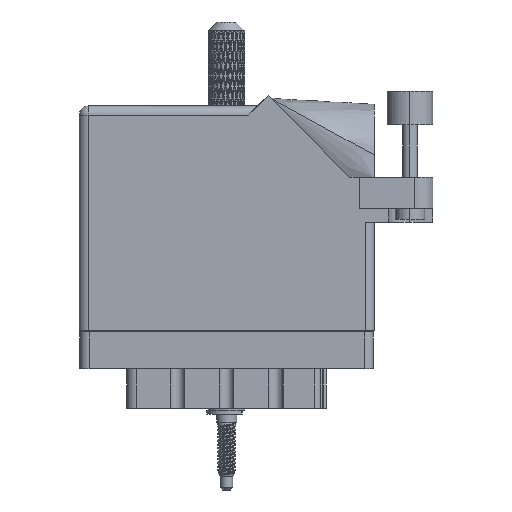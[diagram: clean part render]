
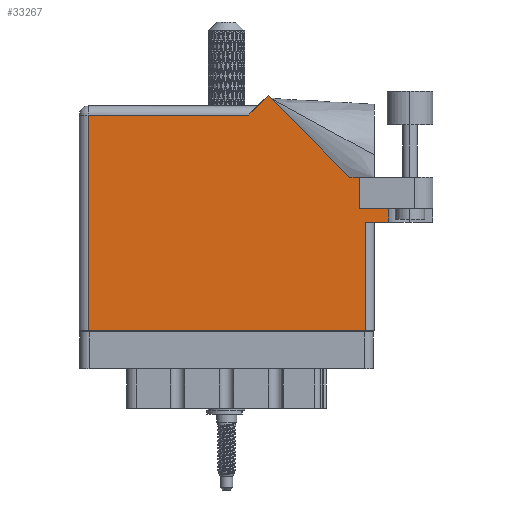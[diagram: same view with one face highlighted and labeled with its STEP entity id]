
A CAD part, front view. The second image highlights one B-rep face of the part: STEP entity #33267.
In plain terms, the highlighted face is planar.
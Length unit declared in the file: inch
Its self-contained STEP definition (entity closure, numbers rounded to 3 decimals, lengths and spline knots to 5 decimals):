
#1179 = FACE_OUTER_BOUND ( 'NONE', #18269, .T. ) ;
#2313 = VERTEX_POINT ( 'NONE', #89890 ) ;
#4279 = EDGE_CURVE ( 'NONE', #44404, #7908, #83758, .T. ) ;
#4425 = EDGE_CURVE ( 'NONE', #72469, #58199, #65546, .T. ) ;
#4754 = CARTESIAN_POINT ( 'NONE',  ( 1.91, 1.044, 0. ) ) ;
#7340 = ORIENTED_EDGE ( 'NONE', *, *, #96079, .T. ) ;
#7737 = EDGE_CURVE ( 'NONE', #39307, #41077, #88404, .T. ) ;
#7908 = VERTEX_POINT ( 'NONE', #36448 ) ;
#8182 = DIRECTION ( 'NONE',  ( -0.707, 0.707, 0. ) ) ;
#10214 = VERTEX_POINT ( 'NONE', #67415 ) ;
#15697 = LINE ( 'NONE', #27255, #35197 ) ;
#16125 = CARTESIAN_POINT ( 'NONE',  ( 1.84442, 1.044, 0. ) ) ;
#16187 = ORIENTED_EDGE ( 'NONE', *, *, #77938, .T. ) ;
#16701 = LINE ( 'NONE', #39897, #78989 ) ;
#18269 = EDGE_LOOP ( 'NONE', ( #16187, #7340, #90625, #33414, #62590, #101086, #53317, #51466, #72402, #36163, #60569 ) ) ;
#18594 = CARTESIAN_POINT ( 'NONE',  ( 1.91, 0.831, 0. ) ) ;
#19756 = VECTOR ( 'NONE', #8182, 39.37008 ) ;
#22445 = VECTOR ( 'NONE', #92384, 39.37008 ) ;
#25556 = EDGE_CURVE ( 'NONE', #72469, #82461, #66177, .T. ) ;
#27255 = CARTESIAN_POINT ( 'NONE',  ( 1.217, 1.53, 0. ) ) ;
#31715 = CARTESIAN_POINT ( 'NONE',  ( 2.01, 0.737, 0. ) ) ;
#31770 = VECTOR ( 'NONE', #35194, 39.37008 ) ;
#32326 = CARTESIAN_POINT ( 'NONE',  ( 2.1115, 0.831, 0. ) ) ;
#33267 = ADVANCED_FACE ( 'NONE', ( #1179 ), #75934, .F. ) ;
#33414 = ORIENTED_EDGE ( 'NONE', *, *, #39408, .F. ) ;
#33597 = DIRECTION ( 'NONE',  ( 0., 0., -1. ) ) ;
#33825 = DIRECTION ( 'NONE',  ( -0.707, -0.707, 0. ) ) ;
#35193 = CARTESIAN_POINT ( 'NONE',  ( 1.948, 0., 0. ) ) ;
#35194 = DIRECTION ( 'NONE',  ( -1., 0., 0. ) ) ;
#35197 = VECTOR ( 'NONE', #33825, 39.37008 ) ;
#36163 = ORIENTED_EDGE ( 'NONE', *, *, #59372, .T. ) ;
#36448 = CARTESIAN_POINT ( 'NONE',  ( 2.1115, 0.737, 0. ) ) ;
#37202 = CARTESIAN_POINT ( 'NONE',  ( 1.155, 1.468, 0. ) ) ;
#39307 = VERTEX_POINT ( 'NONE', #72629 ) ;
#39408 = EDGE_CURVE ( 'NONE', #58199, #7908, #78262, .T. ) ;
#39597 = LINE ( 'NONE', #68829, #31770 ) ;
#39897 = CARTESIAN_POINT ( 'NONE',  ( 2.41, 1.044, 0. ) ) ;
#41077 = VERTEX_POINT ( 'NONE', #67857 ) ;
#41596 = DIRECTION ( 'NONE',  ( -1., 0., 0. ) ) ;
#42699 = VECTOR ( 'NONE', #56760, 39.37008 ) ;
#44404 = VERTEX_POINT ( 'NONE', #84426 ) ;
#45379 = LINE ( 'NONE', #105221, #42699 ) ;
#50594 = CARTESIAN_POINT ( 'NONE',  ( 0., 1.53, 0. ) ) ;
#51466 = ORIENTED_EDGE ( 'NONE', *, *, #7737, .T. ) ;
#51524 = LINE ( 'NONE', #56042, #76130 ) ;
#53317 = ORIENTED_EDGE ( 'NONE', *, *, #82004, .T. ) ;
#56042 = CARTESIAN_POINT ( 'NONE',  ( 0.062, 0., 0. ) ) ;
#56760 = DIRECTION ( 'NONE',  ( 0., 1., 0. ) ) ;
#58199 = VERTEX_POINT ( 'NONE', #32326 ) ;
#58881 = VERTEX_POINT ( 'NONE', #37202 ) ;
#59372 = EDGE_CURVE ( 'NONE', #58881, #10214, #39597, .T. ) ;
#60569 = ORIENTED_EDGE ( 'NONE', *, *, #94367, .T. ) ;
#62590 = ORIENTED_EDGE ( 'NONE', *, *, #4425, .F. ) ;
#64993 = DIRECTION ( 'NONE',  ( 1., 0., 0. ) ) ;
#65154 = DIRECTION ( 'NONE',  ( -1., 0., 0. ) ) ;
#65546 = LINE ( 'NONE', #91689, #100546 ) ;
#66177 = LINE ( 'NONE', #18594, #97239 ) ;
#67415 = CARTESIAN_POINT ( 'NONE',  ( 0.062, 1.468, 0. ) ) ;
#67857 = CARTESIAN_POINT ( 'NONE',  ( 1.28771, 1.60071, 0. ) ) ;
#68829 = CARTESIAN_POINT ( 'NONE',  ( 0., 1.468, 0. ) ) ;
#69188 = CARTESIAN_POINT ( 'NONE',  ( 1.91, 0.831, 0. ) ) ;
#69263 = DIRECTION ( 'NONE',  ( 1., 0., 0. ) ) ;
#70578 = LINE ( 'NONE', #93438, #84782 ) ;
#72402 = ORIENTED_EDGE ( 'NONE', *, *, #90286, .T. ) ;
#72469 = VERTEX_POINT ( 'NONE', #69188 ) ;
#72629 = CARTESIAN_POINT ( 'NONE',  ( 1.84442, 1.044, 0. ) ) ;
#74715 = VECTOR ( 'NONE', #64993, 39.37008 ) ;
#75934 = PLANE ( 'NONE',  #96126 ) ;
#76130 = VECTOR ( 'NONE', #97968, 39.37008 ) ;
#77938 = EDGE_CURVE ( 'NONE', #2313, #101488, #70578, .T. ) ;
#78262 = LINE ( 'NONE', #92024, #22445 ) ;
#78989 = VECTOR ( 'NONE', #65154, 39.37008 ) ;
#82004 = EDGE_CURVE ( 'NONE', #82461, #39307, #16701, .T. ) ;
#82461 = VERTEX_POINT ( 'NONE', #4754 ) ;
#83758 = LINE ( 'NONE', #31715, #74715 ) ;
#84426 = CARTESIAN_POINT ( 'NONE',  ( 1.948, 0.737, 0. ) ) ;
#84782 = VECTOR ( 'NONE', #69263, 39.37008 ) ;
#88404 = LINE ( 'NONE', #16125, #19756 ) ;
#89890 = CARTESIAN_POINT ( 'NONE',  ( 0.062, 0., 0. ) ) ;
#90286 = EDGE_CURVE ( 'NONE', #41077, #58881, #15697, .T. ) ;
#90625 = ORIENTED_EDGE ( 'NONE', *, *, #4279, .T. ) ;
#91689 = CARTESIAN_POINT ( 'NONE',  ( 1.91, 0.831, 0. ) ) ;
#92024 = CARTESIAN_POINT ( 'NONE',  ( 2.1115, 1.16177, 0. ) ) ;
#92056 = DIRECTION ( 'NONE',  ( 0., 1., 0. ) ) ;
#92384 = DIRECTION ( 'NONE',  ( 0., -1., 0. ) ) ;
#93438 = CARTESIAN_POINT ( 'NONE',  ( 0., 0., 0. ) ) ;
#94367 = EDGE_CURVE ( 'NONE', #10214, #2313, #51524, .T. ) ;
#96079 = EDGE_CURVE ( 'NONE', #101488, #44404, #45379, .T. ) ;
#96126 = AXIS2_PLACEMENT_3D ( 'NONE', #50594, #33597, #41596 ) ;
#97239 = VECTOR ( 'NONE', #92056, 39.37008 ) ;
#97968 = DIRECTION ( 'NONE',  ( 0., -1., 0. ) ) ;
#100546 = VECTOR ( 'NONE', #104225, 39.37008 ) ;
#101086 = ORIENTED_EDGE ( 'NONE', *, *, #25556, .T. ) ;
#101488 = VERTEX_POINT ( 'NONE', #35193 ) ;
#104225 = DIRECTION ( 'NONE',  ( 1., 0., 0. ) ) ;
#105221 = CARTESIAN_POINT ( 'NONE',  ( 1.948, 0.737, 0. ) ) ;
